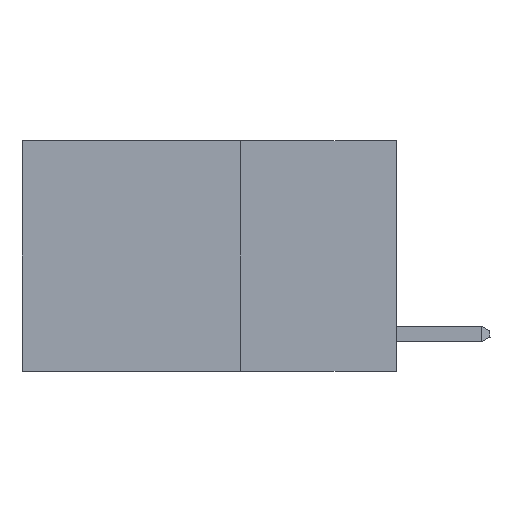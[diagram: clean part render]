
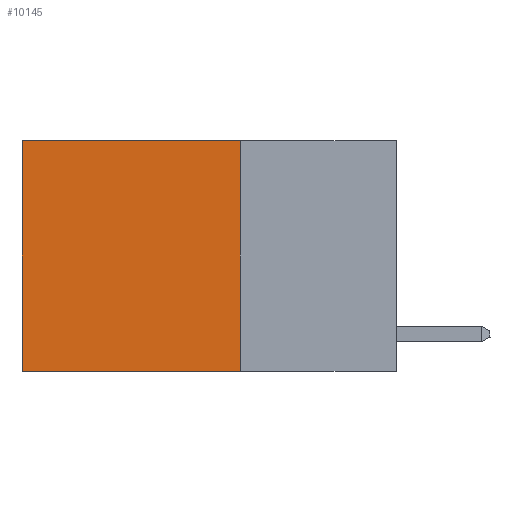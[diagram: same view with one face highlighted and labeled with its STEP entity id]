
A CAD part, left-side view. The second image highlights one B-rep face of the part: STEP entity #10145.
In plain terms, the highlighted planar face has unit normal (-1, 0, 0).
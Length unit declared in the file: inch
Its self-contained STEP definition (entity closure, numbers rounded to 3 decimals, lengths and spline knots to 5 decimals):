
#38 = DIRECTION ( 'NONE',  ( 0., 0., -1. ) ) ;
#90 = VERTEX_POINT ( 'NONE', #6217 ) ;
#174 = CARTESIAN_POINT ( 'NONE',  ( 0.2625, 0.25, -0.37 ) ) ;
#269 = LINE ( 'NONE', #8300, #9113 ) ;
#831 = DIRECTION ( 'NONE',  ( 1., 0., 0. ) ) ;
#1173 = DIRECTION ( 'NONE',  ( 0., 0., -1. ) ) ;
#1431 = CARTESIAN_POINT ( 'NONE',  ( 0.2625, 0.25, 0. ) ) ;
#1759 = VERTEX_POINT ( 'NONE', #7133 ) ;
#2001 = VECTOR ( 'NONE', #9101, 39.37008 ) ;
#2448 = LINE ( 'NONE', #7987, #3629 ) ;
#2881 = LINE ( 'NONE', #3710, #4855 ) ;
#3139 = CARTESIAN_POINT ( 'NONE',  ( 0.2625, 0.6, 0. ) ) ;
#3222 = VERTEX_POINT ( 'NONE', #8073 ) ;
#3629 = VECTOR ( 'NONE', #9665, 39.37008 ) ;
#3662 = ORIENTED_EDGE ( 'NONE', *, *, #7969, .T. ) ;
#3710 = CARTESIAN_POINT ( 'NONE',  ( 0.2625, 0.25, 0. ) ) ;
#4180 = ORIENTED_EDGE ( 'NONE', *, *, #8080, .T. ) ;
#4455 = EDGE_LOOP ( 'NONE', ( #4180, #9840, #10093, #3662 ) ) ;
#4495 = VERTEX_POINT ( 'NONE', #3139 ) ;
#4855 = VECTOR ( 'NONE', #1173, 39.37008 ) ;
#5595 = EDGE_CURVE ( 'NONE', #3222, #90, #2881, .T. ) ;
#5633 = PLANE ( 'NONE',  #9281 ) ;
#5951 = EDGE_CURVE ( 'NONE', #90, #1759, #8933, .T. ) ;
#6217 = CARTESIAN_POINT ( 'NONE',  ( 0.2625, 0.25, -0.37 ) ) ;
#6660 = DIRECTION ( 'NONE',  ( 0., 0., -1. ) ) ;
#7133 = CARTESIAN_POINT ( 'NONE',  ( 0.2625, 0.6, -0.37 ) ) ;
#7969 = EDGE_CURVE ( 'NONE', #3222, #4495, #2448, .T. ) ;
#7987 = CARTESIAN_POINT ( 'NONE',  ( 0.2625, 0.25, 0. ) ) ;
#8073 = CARTESIAN_POINT ( 'NONE',  ( 0.2625, 0.25, 0. ) ) ;
#8080 = EDGE_CURVE ( 'NONE', #4495, #1759, #269, .T. ) ;
#8300 = CARTESIAN_POINT ( 'NONE',  ( 0.2625, 0.6, 0. ) ) ;
#8900 = FACE_OUTER_BOUND ( 'NONE', #4455, .T. ) ;
#8933 = LINE ( 'NONE', #174, #2001 ) ;
#9101 = DIRECTION ( 'NONE',  ( 0., 1., 0. ) ) ;
#9113 = VECTOR ( 'NONE', #6660, 39.37008 ) ;
#9281 = AXIS2_PLACEMENT_3D ( 'NONE', #1431, #831, #38 ) ;
#9665 = DIRECTION ( 'NONE',  ( 0., 1., 0. ) ) ;
#9840 = ORIENTED_EDGE ( 'NONE', *, *, #5951, .F. ) ;
#10093 = ORIENTED_EDGE ( 'NONE', *, *, #5595, .F. ) ;
#10145 = ADVANCED_FACE ( 'NONE', ( #8900 ), #5633, .F. ) ;
